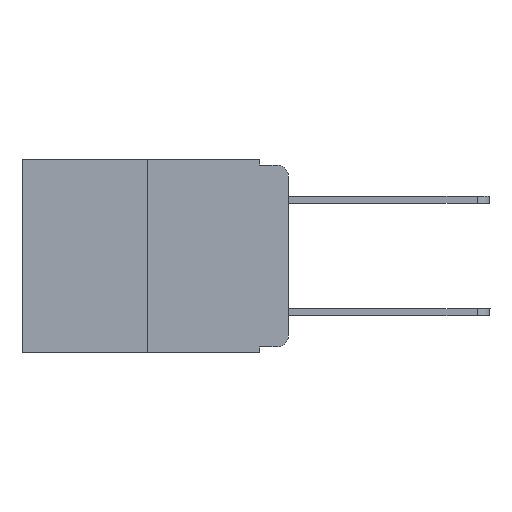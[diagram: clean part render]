
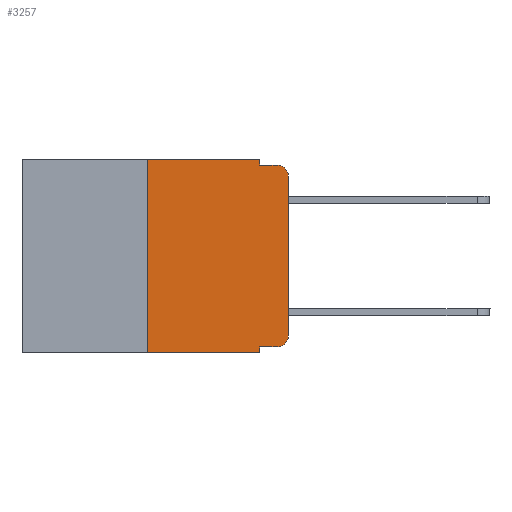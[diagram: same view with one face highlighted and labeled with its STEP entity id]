
A CAD part, left-side view. The second image highlights one B-rep face of the part: STEP entity #3257.
In plain terms, the highlighted planar face has unit normal (-1, 0, 0).
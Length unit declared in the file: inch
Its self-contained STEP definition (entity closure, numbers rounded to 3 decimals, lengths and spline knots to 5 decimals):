
#129 = CARTESIAN_POINT ( 'NONE',  ( 0., 0.02, -0.01 ) ) ;
#132 = CARTESIAN_POINT ( 'NONE',  ( 0., 0.02, -0.313 ) ) ;
#301 = EDGE_CURVE ( 'NONE', #923, #6181, #2097, .T. ) ;
#465 = VECTOR ( 'NONE', #6946, 39.37008 ) ;
#556 = EDGE_CURVE ( 'NONE', #9790, #7236, #8021, .T. ) ;
#557 = ORIENTED_EDGE ( 'NONE', *, *, #4577, .T. ) ;
#618 = EDGE_CURVE ( 'NONE', #1307, #9713, #10151, .T. ) ;
#823 = EDGE_CURVE ( 'NONE', #9229, #8514, #2073, .T. ) ;
#913 = ORIENTED_EDGE ( 'NONE', *, *, #3584, .F. ) ;
#923 = VERTEX_POINT ( 'NONE', #4259 ) ;
#1136 = EDGE_CURVE ( 'NONE', #6181, #9944, #6832, .T. ) ;
#1307 = VERTEX_POINT ( 'NONE', #8334 ) ;
#1364 = CARTESIAN_POINT ( 'NONE',  ( 0., 0.02, -0.03 ) ) ;
#1580 = CARTESIAN_POINT ( 'NONE',  ( 0., 0.25, 0. ) ) ;
#1824 = ORIENTED_EDGE ( 'NONE', *, *, #7138, .T. ) ;
#2073 = LINE ( 'NONE', #5385, #6194 ) ;
#2097 = LINE ( 'NONE', #2207, #8304 ) ;
#2207 = CARTESIAN_POINT ( 'NONE',  ( 0., 0.25, 0. ) ) ;
#2454 = DIRECTION ( 'NONE',  ( 0., -1., 0. ) ) ;
#2662 = AXIS2_PLACEMENT_3D ( 'NONE', #132, #7043, #8732 ) ;
#2816 = EDGE_CURVE ( 'NONE', #9229, #5772, #3273, .T. ) ;
#2855 = ORIENTED_EDGE ( 'NONE', *, *, #618, .T. ) ;
#3257 = ADVANCED_FACE ( 'NONE', ( #6544 ), #7954, .F. ) ;
#3273 = LINE ( 'NONE', #3341, #465 ) ;
#3341 = CARTESIAN_POINT ( 'NONE',  ( 0., 0.051, 0. ) ) ;
#3498 = CARTESIAN_POINT ( 'NONE',  ( 0., 0.051, -0.343 ) ) ;
#3584 = EDGE_CURVE ( 'NONE', #9944, #9790, #8104, .T. ) ;
#3715 = CARTESIAN_POINT ( 'NONE',  ( 0., 0.051, 0. ) ) ;
#3770 = DIRECTION ( 'NONE',  ( 1., 0., 0. ) ) ;
#4259 = CARTESIAN_POINT ( 'NONE',  ( 0., 0.25, -0.343 ) ) ;
#4555 = CARTESIAN_POINT ( 'NONE',  ( 0., 0.473, 0. ) ) ;
#4577 = EDGE_CURVE ( 'NONE', #8514, #1307, #4655, .T. ) ;
#4611 = DIRECTION ( 'NONE',  ( 0., 0., 1. ) ) ;
#4628 = AXIS2_PLACEMENT_3D ( 'NONE', #10398, #3770, #5466 ) ;
#4650 = AXIS2_PLACEMENT_3D ( 'NONE', #1364, #7284, #8002 ) ;
#4655 = CIRCLE ( 'NONE', #2662, 0.02 ) ;
#4860 = CARTESIAN_POINT ( 'NONE',  ( 0., 0.051, -0.01 ) ) ;
#4908 = ORIENTED_EDGE ( 'NONE', *, *, #556, .F. ) ;
#5289 = CARTESIAN_POINT ( 'NONE',  ( 0., 0.02, -0.333 ) ) ;
#5385 = CARTESIAN_POINT ( 'NONE',  ( 0., 0.051, -0.333 ) ) ;
#5466 = DIRECTION ( 'NONE',  ( 0., 0., -1. ) ) ;
#5506 = DIRECTION ( 'NONE',  ( 0., -1., 0. ) ) ;
#5523 = DIRECTION ( 'NONE',  ( 0., 0., -1. ) ) ;
#5601 = ORIENTED_EDGE ( 'NONE', *, *, #2816, .F. ) ;
#5772 = VERTEX_POINT ( 'NONE', #3498 ) ;
#5978 = EDGE_CURVE ( 'NONE', #9713, #7236, #9170, .T. ) ;
#6015 = ORIENTED_EDGE ( 'NONE', *, *, #1136, .F. ) ;
#6049 = ORIENTED_EDGE ( 'NONE', *, *, #823, .T. ) ;
#6181 = VERTEX_POINT ( 'NONE', #1580 ) ;
#6194 = VECTOR ( 'NONE', #6278, 39.37008 ) ;
#6268 = VECTOR ( 'NONE', #2454, 39.37008 ) ;
#6278 = DIRECTION ( 'NONE',  ( 0., -1., 0. ) ) ;
#6331 = VECTOR ( 'NONE', #7405, 39.37008 ) ;
#6509 = CARTESIAN_POINT ( 'NONE',  ( 0., 0., 0. ) ) ;
#6544 = FACE_OUTER_BOUND ( 'NONE', #8032, .T. ) ;
#6832 = LINE ( 'NONE', #4555, #7382 ) ;
#6848 = VECTOR ( 'NONE', #9551, 39.37008 ) ;
#6924 = VECTOR ( 'NONE', #5523, 39.37008 ) ;
#6942 = CARTESIAN_POINT ( 'NONE',  ( 0., 0., -0.03 ) ) ;
#6946 = DIRECTION ( 'NONE',  ( 0., 0., -1. ) ) ;
#7043 = DIRECTION ( 'NONE',  ( -1., 0., 0. ) ) ;
#7138 = EDGE_CURVE ( 'NONE', #923, #5772, #8091, .T. ) ;
#7236 = VERTEX_POINT ( 'NONE', #129 ) ;
#7250 = CARTESIAN_POINT ( 'NONE',  ( 0., 0.051, -0.333 ) ) ;
#7284 = DIRECTION ( 'NONE',  ( -1., 0., 0. ) ) ;
#7382 = VECTOR ( 'NONE', #5506, 39.37008 ) ;
#7405 = DIRECTION ( 'NONE',  ( 0., -1., 0. ) ) ;
#7954 = PLANE ( 'NONE',  #4628 ) ;
#8002 = DIRECTION ( 'NONE',  ( 0., 0., -1. ) ) ;
#8021 = LINE ( 'NONE', #4860, #6331 ) ;
#8032 = EDGE_LOOP ( 'NONE', ( #2855, #8437, #4908, #913, #6015, #9375, #1824, #5601, #6049, #557 ) ) ;
#8091 = LINE ( 'NONE', #10809, #6268 ) ;
#8104 = LINE ( 'NONE', #9682, #6924 ) ;
#8304 = VECTOR ( 'NONE', #4611, 39.37008 ) ;
#8334 = CARTESIAN_POINT ( 'NONE',  ( 0., 0., -0.313 ) ) ;
#8437 = ORIENTED_EDGE ( 'NONE', *, *, #5978, .T. ) ;
#8514 = VERTEX_POINT ( 'NONE', #5289 ) ;
#8732 = DIRECTION ( 'NONE',  ( 0., 0., -1. ) ) ;
#9170 = CIRCLE ( 'NONE', #4650, 0.02 ) ;
#9229 = VERTEX_POINT ( 'NONE', #7250 ) ;
#9375 = ORIENTED_EDGE ( 'NONE', *, *, #301, .F. ) ;
#9551 = DIRECTION ( 'NONE',  ( 0., 0., 1. ) ) ;
#9561 = CARTESIAN_POINT ( 'NONE',  ( 0., 0.051, -0.01 ) ) ;
#9682 = CARTESIAN_POINT ( 'NONE',  ( 0., 0.051, 0. ) ) ;
#9713 = VERTEX_POINT ( 'NONE', #6942 ) ;
#9790 = VERTEX_POINT ( 'NONE', #9561 ) ;
#9944 = VERTEX_POINT ( 'NONE', #3715 ) ;
#10151 = LINE ( 'NONE', #6509, #6848 ) ;
#10398 = CARTESIAN_POINT ( 'NONE',  ( 0., 0.473, 0. ) ) ;
#10809 = CARTESIAN_POINT ( 'NONE',  ( 0., 0.473, -0.343 ) ) ;
